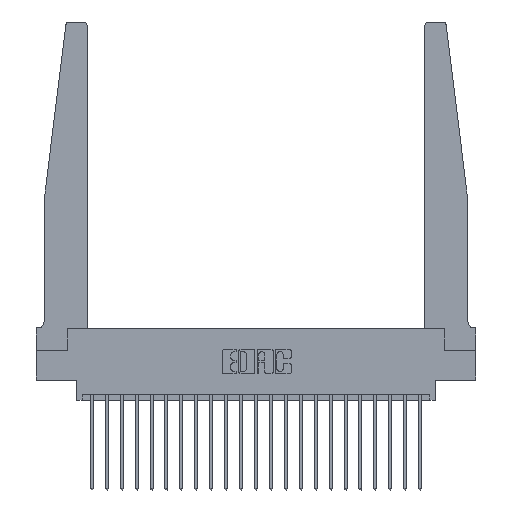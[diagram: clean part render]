
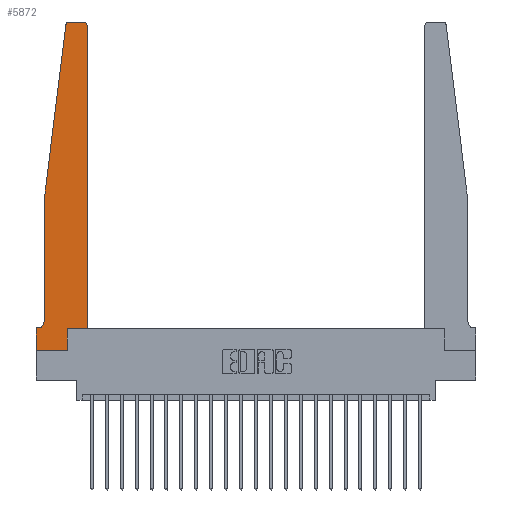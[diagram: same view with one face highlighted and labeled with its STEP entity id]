
A CAD part, top view. The second image highlights one B-rep face of the part: STEP entity #5872.
In plain terms, the highlighted planar face has unit normal (0, 0, 1).
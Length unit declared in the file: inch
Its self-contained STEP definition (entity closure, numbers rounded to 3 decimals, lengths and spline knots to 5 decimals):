
#61 = ORIENTED_EDGE ( 'NONE', *, *, #9068, .T. ) ;
#825 = EDGE_CURVE ( 'NONE', #18896, #16173, #18951, .T. ) ;
#1120 = CARTESIAN_POINT ( 'NONE',  ( 0., 0., 0.37 ) ) ;
#1291 = ORIENTED_EDGE ( 'NONE', *, *, #18024, .T. ) ;
#1949 = ORIENTED_EDGE ( 'NONE', *, *, #17102, .T. ) ;
#2037 = VERTEX_POINT ( 'NONE', #18068 ) ;
#2093 = ORIENTED_EDGE ( 'NONE', *, *, #2589, .T. ) ;
#2425 = VECTOR ( 'NONE', #6617, 39.37008 ) ;
#2580 = DIRECTION ( 'NONE',  ( 0., 0., 1. ) ) ;
#2589 = EDGE_CURVE ( 'NONE', #8904, #18896, #10537, .T. ) ;
#2605 = VERTEX_POINT ( 'NONE', #19930 ) ;
#2673 = EDGE_LOOP ( 'NONE', ( #6318, #7262, #1291, #2093, #6536, #10326, #4547, #5804, #61, #1949, #21734, #15417 ) ) ;
#2701 = DIRECTION ( 'NONE',  ( 1., 0., 0. ) ) ;
#2866 = DIRECTION ( 'NONE',  ( 0., -1., 0. ) ) ;
#3052 = LINE ( 'NONE', #4373, #16405 ) ;
#3261 = DIRECTION ( 'NONE',  ( -1., 0., 0. ) ) ;
#3869 = CARTESIAN_POINT ( 'NONE',  ( 0.395, 2.75, 0.37 ) ) ;
#4100 = VERTEX_POINT ( 'NONE', #8662 ) ;
#4373 = CARTESIAN_POINT ( 'NONE',  ( 0.425, 0.18, 0.37 ) ) ;
#4485 = VECTOR ( 'NONE', #2866, 39.37008 ) ;
#4547 = ORIENTED_EDGE ( 'NONE', *, *, #12186, .T. ) ;
#4890 = CARTESIAN_POINT ( 'NONE',  ( 0.2605, 0.18, 0.37 ) ) ;
#5035 = CARTESIAN_POINT ( 'NONE',  ( 0.425, 0.18, 0.37 ) ) ;
#5072 = DIRECTION ( 'NONE',  ( 0., 0., 1. ) ) ;
#5804 = ORIENTED_EDGE ( 'NONE', *, *, #11257, .T. ) ;
#5872 = ADVANCED_FACE ( 'NONE', ( #6082 ), #22403, .T. ) ;
#5927 = LINE ( 'NONE', #5035, #14681 ) ;
#5992 = CARTESIAN_POINT ( 'NONE',  ( 0.065, 1.25, 0.37 ) ) ;
#6082 = FACE_OUTER_BOUND ( 'NONE', #2673, .T. ) ;
#6318 = ORIENTED_EDGE ( 'NONE', *, *, #12312, .T. ) ;
#6536 = ORIENTED_EDGE ( 'NONE', *, *, #825, .T. ) ;
#6617 = DIRECTION ( 'NONE',  ( 0., 1., 0. ) ) ;
#6778 = DIRECTION ( 'NONE',  ( 0., 1., 0. ) ) ;
#6864 = VERTEX_POINT ( 'NONE', #10099 ) ;
#7262 = ORIENTED_EDGE ( 'NONE', *, *, #19111, .T. ) ;
#8208 = AXIS2_PLACEMENT_3D ( 'NONE', #13756, #5072, #17264 ) ;
#8289 = VECTOR ( 'NONE', #21091, 39.37008 ) ;
#8662 = CARTESIAN_POINT ( 'NONE',  ( 0.2605, 0.18, 0.37 ) ) ;
#8747 = DIRECTION ( 'NONE',  ( -0.122, -0.992, 0. ) ) ;
#8895 = DIRECTION ( 'NONE',  ( 0., 0., 1. ) ) ;
#8904 = VERTEX_POINT ( 'NONE', #16558 ) ;
#8921 = CARTESIAN_POINT ( 'NONE',  ( 0., 0., 0.37 ) ) ;
#9068 = EDGE_CURVE ( 'NONE', #13776, #4100, #11616, .T. ) ;
#9140 = EDGE_CURVE ( 'NONE', #13680, #10030, #5927, .T. ) ;
#9330 = CARTESIAN_POINT ( 'NONE',  ( 0.425, 2.72, 0.37 ) ) ;
#9345 = CARTESIAN_POINT ( 'NONE',  ( 0.015, 0.2375, 0.37 ) ) ;
#10030 = VERTEX_POINT ( 'NONE', #9330 ) ;
#10099 = CARTESIAN_POINT ( 'NONE',  ( 0.27653, 2.75, 0.37 ) ) ;
#10326 = ORIENTED_EDGE ( 'NONE', *, *, #11083, .T. ) ;
#10537 = LINE ( 'NONE', #5992, #20357 ) ;
#10983 = VECTOR ( 'NONE', #11879, 39.37008 ) ;
#11064 = DIRECTION ( 'NONE',  ( -1., 0., 0. ) ) ;
#11083 = EDGE_CURVE ( 'NONE', #16173, #2037, #11524, .T. ) ;
#11205 = CIRCLE ( 'NONE', #13825, 0.03 ) ;
#11257 = EDGE_CURVE ( 'NONE', #12126, #13776, #17045, .T. ) ;
#11524 = LINE ( 'NONE', #18916, #10983 ) ;
#11616 = LINE ( 'NONE', #4890, #2425 ) ;
#11879 = DIRECTION ( 'NONE',  ( -1., 0., 0. ) ) ;
#12082 = CARTESIAN_POINT ( 'NONE',  ( 0.015, 0.1875, 0.37 ) ) ;
#12126 = VERTEX_POINT ( 'NONE', #18116 ) ;
#12186 = EDGE_CURVE ( 'NONE', #2037, #12126, #13757, .T. ) ;
#12312 = EDGE_CURVE ( 'NONE', #21620, #6864, #20816, .T. ) ;
#12744 = CARTESIAN_POINT ( 'NONE',  ( 0.425, 0.18, 0.37 ) ) ;
#12807 = VECTOR ( 'NONE', #8747, 39.37008 ) ;
#12991 = CARTESIAN_POINT ( 'NONE',  ( 0.2605, 0., 0.37 ) ) ;
#13016 = CARTESIAN_POINT ( 'NONE',  ( 0.395, 2.72, 0.37 ) ) ;
#13085 = EDGE_CURVE ( 'NONE', #10030, #21620, #11205, .T. ) ;
#13354 = LINE ( 'NONE', #20920, #12807 ) ;
#13680 = VERTEX_POINT ( 'NONE', #12744 ) ;
#13756 = CARTESIAN_POINT ( 'NONE',  ( 0., 0.1875, 0.37 ) ) ;
#13757 = LINE ( 'NONE', #1120, #4485 ) ;
#13776 = VERTEX_POINT ( 'NONE', #12991 ) ;
#13825 = AXIS2_PLACEMENT_3D ( 'NONE', #13016, #2580, #14779 ) ;
#14681 = VECTOR ( 'NONE', #6778, 39.37008 ) ;
#14779 = DIRECTION ( 'NONE',  ( 1., 0., 0. ) ) ;
#15227 = CIRCLE ( 'NONE', #19602, 0.03 ) ;
#15417 = ORIENTED_EDGE ( 'NONE', *, *, #13085, .T. ) ;
#15447 = CARTESIAN_POINT ( 'NONE',  ( 0.25, 2.75, 0.37 ) ) ;
#16173 = VERTEX_POINT ( 'NONE', #12082 ) ;
#16405 = VECTOR ( 'NONE', #2701, 39.37008 ) ;
#16558 = CARTESIAN_POINT ( 'NONE',  ( 0.065, 1.25, 0.37 ) ) ;
#16929 = CARTESIAN_POINT ( 'NONE',  ( 0.065, 0.2375, 0.37 ) ) ;
#17045 = LINE ( 'NONE', #8921, #8289 ) ;
#17102 = EDGE_CURVE ( 'NONE', #4100, #13680, #3052, .T. ) ;
#17264 = DIRECTION ( 'NONE',  ( 1., 0., 0. ) ) ;
#18024 = EDGE_CURVE ( 'NONE', #2605, #8904, #13354, .T. ) ;
#18068 = CARTESIAN_POINT ( 'NONE',  ( 0., 0.1875, 0.37 ) ) ;
#18116 = CARTESIAN_POINT ( 'NONE',  ( 0., 0., 0.37 ) ) ;
#18189 = DIRECTION ( 'NONE',  ( 0., -1., 0. ) ) ;
#18896 = VERTEX_POINT ( 'NONE', #16929 ) ;
#18916 = CARTESIAN_POINT ( 'NONE',  ( 0.065, 0.1875, 0.37 ) ) ;
#18951 = CIRCLE ( 'NONE', #20983, 0.05 ) ;
#19111 = EDGE_CURVE ( 'NONE', #6864, #2605, #15227, .T. ) ;
#19345 = CARTESIAN_POINT ( 'NONE',  ( 0.27653, 2.72, 0.37 ) ) ;
#19602 = AXIS2_PLACEMENT_3D ( 'NONE', #19345, #8895, #21059 ) ;
#19930 = CARTESIAN_POINT ( 'NONE',  ( 0.24675, 2.72367, 0.37 ) ) ;
#20357 = VECTOR ( 'NONE', #18189, 39.37008 ) ;
#20816 = LINE ( 'NONE', #15447, #21348 ) ;
#20920 = CARTESIAN_POINT ( 'NONE',  ( 0.065, 1.25, 0.37 ) ) ;
#20983 = AXIS2_PLACEMENT_3D ( 'NONE', #9345, #21533, #11064 ) ;
#21059 = DIRECTION ( 'NONE',  ( 1., 0., 0. ) ) ;
#21091 = DIRECTION ( 'NONE',  ( 1., 0., 0. ) ) ;
#21348 = VECTOR ( 'NONE', #3261, 39.37008 ) ;
#21533 = DIRECTION ( 'NONE',  ( 0., 0., -1. ) ) ;
#21620 = VERTEX_POINT ( 'NONE', #3869 ) ;
#21734 = ORIENTED_EDGE ( 'NONE', *, *, #9140, .T. ) ;
#22403 = PLANE ( 'NONE',  #8208 ) ;
